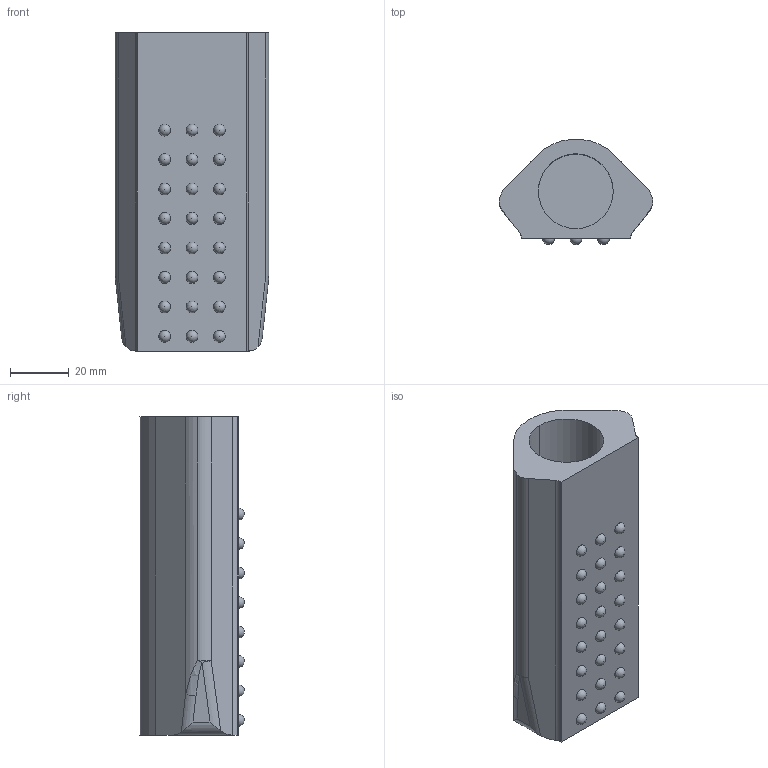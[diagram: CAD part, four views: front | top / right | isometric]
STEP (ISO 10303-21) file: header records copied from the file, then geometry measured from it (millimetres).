
FILE_DESCRIPTION (( 'STEP AP214' ), '1' );
FILE_NAME ('Buffer_Tube_2b.STEP', '2013-09-01T16:37:54', ( 'Asher' ), ( '' ), 'SwSTEP 2.0', 'SolidWorks 2013', '' );
FILE_SCHEMA (( 'AUTOMOTIVE_DESIGN' ));
Length unit declared in the file: millimetre
Products named in the file (1): Buffer_Tube_2b
Bounding box: 52.09 x 35.59 x 108 mm (x, y, z)
Volume: 96387.4 mm3; surface area: 24702.5 mm2
Topology: 1 solids, 1 shells, 56 faces, 199 edges, 146 vertices
Faces by surface type: sphere 26, cylinder 16, plane 12, bspline 2
Entity records: 1725 total; most frequent: CARTESIAN_POINT 358, DIRECTION 295, ORIENTED_EDGE 254, EDGE_CURVE 127, AXIS2_PLACEMENT_3D 127, VERTEX_POINT 98, EDGE_LOOP 81, CIRCLE 72
